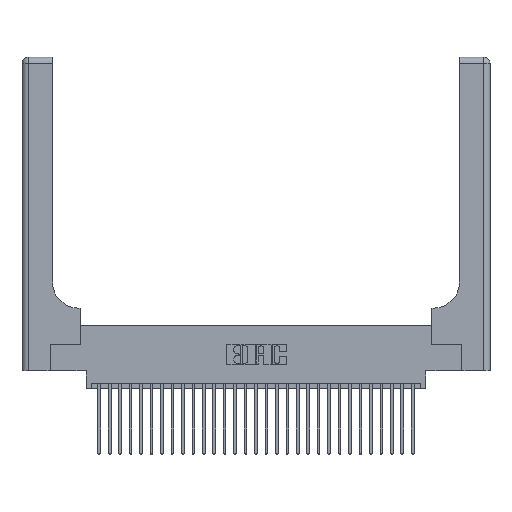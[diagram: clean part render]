
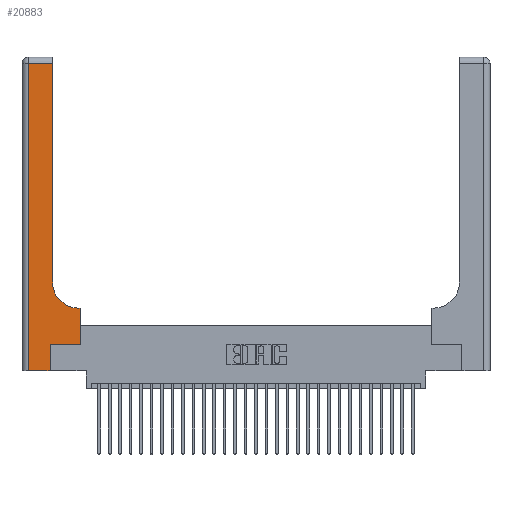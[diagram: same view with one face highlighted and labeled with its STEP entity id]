
A CAD part, top view. The second image highlights one B-rep face of the part: STEP entity #20883.
In plain terms, the highlighted planar face has unit normal (0, 0, 1).
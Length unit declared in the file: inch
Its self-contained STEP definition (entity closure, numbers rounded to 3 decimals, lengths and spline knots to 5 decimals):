
#15 = EDGE_CURVE ( 'NONE', #20495, #4573, #21386, .T. ) ;
#264 = CARTESIAN_POINT ( 'NONE',  ( 0.269, 0., 0.37 ) ) ;
#685 = EDGE_CURVE ( 'NONE', #23925, #23854, #17917, .T. ) ;
#828 = DIRECTION ( 'NONE',  ( 0., 0., -1. ) ) ;
#829 = VECTOR ( 'NONE', #26652, 39.37008 ) ;
#1355 = AXIS2_PLACEMENT_3D ( 'NONE', #3130, #828, #5660 ) ;
#2819 = CARTESIAN_POINT ( 'NONE',  ( 0.2915, 0.6, 0.37 ) ) ;
#2920 = LINE ( 'NONE', #2819, #11205 ) ;
#3079 = CARTESIAN_POINT ( 'NONE',  ( 0.5415, 0.6, 0.37 ) ) ;
#3130 = CARTESIAN_POINT ( 'NONE',  ( 0., 3., 0.37 ) ) ;
#3315 = CARTESIAN_POINT ( 'NONE',  ( 0.06, 3., 0.37 ) ) ;
#3826 = DIRECTION ( 'NONE',  ( -1., 0., 0. ) ) ;
#3987 = ORIENTED_EDGE ( 'NONE', *, *, #24526, .T. ) ;
#4292 = EDGE_CURVE ( 'NONE', #6354, #25675, #19257, .T. ) ;
#4306 = VERTEX_POINT ( 'NONE', #20936 ) ;
#4573 = VERTEX_POINT ( 'NONE', #17265 ) ;
#4732 = EDGE_LOOP ( 'NONE', ( #20652, #6366, #18176, #16911, #3987, #30456, #14442, #5052, #30291 ) ) ;
#5052 = ORIENTED_EDGE ( 'NONE', *, *, #30583, .T. ) ;
#5317 = EDGE_CURVE ( 'NONE', #7344, #4306, #12026, .T. ) ;
#5660 = DIRECTION ( 'NONE',  ( -1., 0., 0. ) ) ;
#5726 = EDGE_CURVE ( 'NONE', #25675, #23925, #30898, .T. ) ;
#5891 = VECTOR ( 'NONE', #3826, 39.37008 ) ;
#6061 = DIRECTION ( 'NONE',  ( 0., -1., 0. ) ) ;
#6354 = VERTEX_POINT ( 'NONE', #3079 ) ;
#6366 = ORIENTED_EDGE ( 'NONE', *, *, #685, .T. ) ;
#6873 = DIRECTION ( 'NONE',  ( 0., 0., -1. ) ) ;
#7186 = CARTESIAN_POINT ( 'NONE',  ( 0.5415, 0.85, 0.37 ) ) ;
#7344 = VERTEX_POINT ( 'NONE', #29024 ) ;
#7590 = DIRECTION ( 'NONE',  ( 1., 0., 0. ) ) ;
#7911 = CARTESIAN_POINT ( 'NONE',  ( 0.5585, 0.25, 0.37 ) ) ;
#8692 = VECTOR ( 'NONE', #6061, 39.37008 ) ;
#10108 = DIRECTION ( 'NONE',  ( 0., 1., 0. ) ) ;
#10382 = DIRECTION ( 'NONE',  ( 0., 1., 0. ) ) ;
#11205 = VECTOR ( 'NONE', #26716, 39.37008 ) ;
#11910 = EDGE_CURVE ( 'NONE', #23854, #20495, #13186, .T. ) ;
#12026 = LINE ( 'NONE', #24812, #28627 ) ;
#12370 = CARTESIAN_POINT ( 'NONE',  ( 0.06, 2.94, 0.37 ) ) ;
#12719 = DIRECTION ( 'NONE',  ( 1., 0., 0. ) ) ;
#12831 = DIRECTION ( 'NONE',  ( 1., 0., 0. ) ) ;
#13186 = LINE ( 'NONE', #3315, #8692 ) ;
#13220 = PLANE ( 'NONE',  #1355 ) ;
#13946 = EDGE_CURVE ( 'NONE', #4306, #17181, #25589, .T. ) ;
#14442 = ORIENTED_EDGE ( 'NONE', *, *, #13946, .T. ) ;
#14797 = CARTESIAN_POINT ( 'NONE',  ( 0., 0., 0.37 ) ) ;
#14959 = VECTOR ( 'NONE', #7590, 39.37008 ) ;
#16904 = VECTOR ( 'NONE', #10382, 39.37008 ) ;
#16911 = ORIENTED_EDGE ( 'NONE', *, *, #15, .T. ) ;
#17181 = VERTEX_POINT ( 'NONE', #30798 ) ;
#17265 = CARTESIAN_POINT ( 'NONE',  ( 0.269, 0., 0.37 ) ) ;
#17917 = LINE ( 'NONE', #30262, #5891 ) ;
#18176 = ORIENTED_EDGE ( 'NONE', *, *, #11910, .T. ) ;
#19257 = CIRCLE ( 'NONE', #22248, 0.25 ) ;
#19434 = CARTESIAN_POINT ( 'NONE',  ( 0.2915, 0.85, 0.37 ) ) ;
#19827 = CARTESIAN_POINT ( 'NONE',  ( 0.2915, 3., 0.37 ) ) ;
#20495 = VERTEX_POINT ( 'NONE', #30842 ) ;
#20652 = ORIENTED_EDGE ( 'NONE', *, *, #5726, .T. ) ;
#20883 = ADVANCED_FACE ( 'NONE', ( #25135 ), #13220, .F. ) ;
#20936 = CARTESIAN_POINT ( 'NONE',  ( 0.5585, 0.25, 0.37 ) ) ;
#21386 = LINE ( 'NONE', #14797, #14959 ) ;
#22248 = AXIS2_PLACEMENT_3D ( 'NONE', #7186, #6873, #12831 ) ;
#23854 = VERTEX_POINT ( 'NONE', #12370 ) ;
#23925 = VERTEX_POINT ( 'NONE', #26910 ) ;
#24526 = EDGE_CURVE ( 'NONE', #4573, #7344, #24906, .T. ) ;
#24812 = CARTESIAN_POINT ( 'NONE',  ( 0.269, 0.25, 0.37 ) ) ;
#24906 = LINE ( 'NONE', #264, #829 ) ;
#25135 = FACE_OUTER_BOUND ( 'NONE', #4732, .T. ) ;
#25589 = LINE ( 'NONE', #7911, #26353 ) ;
#25675 = VERTEX_POINT ( 'NONE', #19434 ) ;
#26353 = VECTOR ( 'NONE', #10108, 39.37008 ) ;
#26652 = DIRECTION ( 'NONE',  ( 0., 1., 0. ) ) ;
#26716 = DIRECTION ( 'NONE',  ( -1., 0., 0. ) ) ;
#26910 = CARTESIAN_POINT ( 'NONE',  ( 0.2915, 2.94, 0.37 ) ) ;
#28627 = VECTOR ( 'NONE', #12719, 39.37008 ) ;
#29024 = CARTESIAN_POINT ( 'NONE',  ( 0.269, 0.25, 0.37 ) ) ;
#30262 = CARTESIAN_POINT ( 'NONE',  ( 0., 2.94, 0.37 ) ) ;
#30291 = ORIENTED_EDGE ( 'NONE', *, *, #4292, .T. ) ;
#30456 = ORIENTED_EDGE ( 'NONE', *, *, #5317, .T. ) ;
#30583 = EDGE_CURVE ( 'NONE', #17181, #6354, #2920, .T. ) ;
#30798 = CARTESIAN_POINT ( 'NONE',  ( 0.5585, 0.6, 0.37 ) ) ;
#30842 = CARTESIAN_POINT ( 'NONE',  ( 0.06, 0., 0.37 ) ) ;
#30898 = LINE ( 'NONE', #19827, #16904 ) ;
